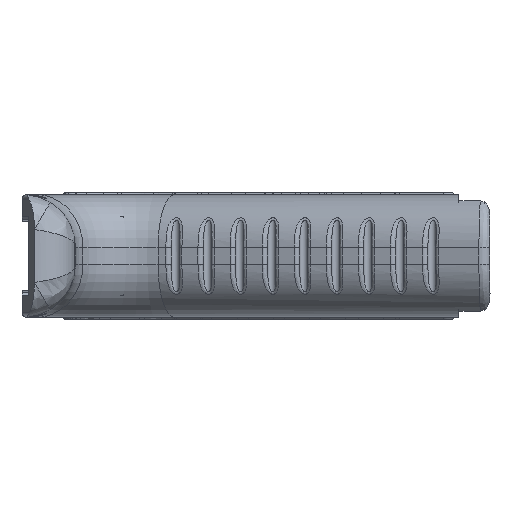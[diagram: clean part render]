
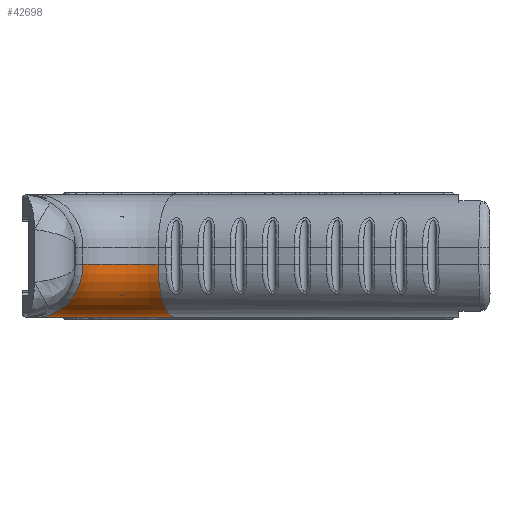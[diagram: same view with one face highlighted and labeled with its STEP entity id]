
A CAD part, left-side view. The second image highlights one B-rep face of the part: STEP entity #42698.
In plain terms, the highlighted toroidal (fillet/blend) face has major radius 27.537 mm and minor radius 12.5 mm.
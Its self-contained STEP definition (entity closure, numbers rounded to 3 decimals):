
#1002=TOROIDAL_SURFACE('',#44390,27.537,12.5);
#1278=B_SPLINE_CURVE_WITH_KNOTS('',3,(#81978,#81979,#81980,#81981,#81982,
#81983,#81984,#81985,#81986,#81987,#81988,#81989,#81990,#81991,#81992,#81993,
#81994,#81995,#81996,#81997,#81998,#81999,#82000,#82001,#82002,#82003,#82004,
#82005,#82006,#82007,#82008,#82009,#82010,#82011,#82012,#82013,#82014,#82015,
#82016,#82017,#82018,#82019,#82020,#82021,#82022,#82023,#82024,#82025,#82026,
#82027,#82028,#82029),.UNSPECIFIED.,.F.,.F.,(4,3,3,3,3,3,3,3,3,3,3,3,3,
3,3,3,3,4),(-0.008,0.,0.131,0.314,
0.448,0.497,0.627,0.806,
0.94,0.985,1.115,1.294,1.429,
1.473,1.604,1.783,1.915,1.961),
 .UNSPECIFIED.);
#3668=CIRCLE('',#43090,27.537);
#3890=CIRCLE('',#44312,15.037);
#3922=CIRCLE('',#44391,12.5);
#6183=FACE_OUTER_BOUND('',#8610,.T.);
#8610=EDGE_LOOP('',(#37997,#37998,#37999,#38000));
#16500=VERTEX_POINT('',#52969);
#16501=VERTEX_POINT('',#52971);
#20166=VERTEX_POINT('',#80456);
#20168=VERTEX_POINT('',#81551);
#20689=EDGE_CURVE('',#16501,#16500,#3668,.T.);
#26236=EDGE_CURVE('',#20166,#20168,#3890,.T.);
#26347=EDGE_CURVE('',#16501,#20168,#1278,.T.);
#26348=EDGE_CURVE('',#20166,#16500,#3922,.T.);
#37997=ORIENTED_EDGE('',*,*,#20689,.T.);
#37998=ORIENTED_EDGE('',*,*,#26348,.F.);
#37999=ORIENTED_EDGE('',*,*,#26236,.T.);
#38000=ORIENTED_EDGE('',*,*,#26347,.F.);
#42698=ADVANCED_FACE('',(#6183),#1002,.T.);
#43090=AXIS2_PLACEMENT_3D('',#52972,#45144,#45145);
#44312=AXIS2_PLACEMENT_3D('',#81552,#50798,#50799);
#44390=AXIS2_PLACEMENT_3D('',#82030,#51021,#51022);
#44391=AXIS2_PLACEMENT_3D('',#82031,#51023,#51024);
#45144=DIRECTION('center_axis',(0.,0.,-1.));
#45145=DIRECTION('ref_axis',(0.93,0.368,0.));
#50798=DIRECTION('center_axis',(0.,0.,1.));
#50799=DIRECTION('ref_axis',(0.93,0.368,0.));
#51021=DIRECTION('center_axis',(0.,0.,1.));
#51022=DIRECTION('ref_axis',(1.,0.,0.));
#51023=DIRECTION('center_axis',(-0.309,-0.951,0.));
#51024=DIRECTION('ref_axis',(-0.951,0.309,0.));
#52969=CARTESIAN_POINT('',(-54.134,133.337,-34.));
#52971=CARTESIAN_POINT('',(-66.871,165.874,-34.));
#52972=CARTESIAN_POINT('Origin',(-80.324,141.847,-34.));
#80456=CARTESIAN_POINT('',(-66.022,137.2,-21.5));
#81551=CARTESIAN_POINT('',(-73.077,155.023,-21.5));
#81552=CARTESIAN_POINT('Origin',(-80.324,141.847,-21.5));
#81978=CARTESIAN_POINT('Ctrl Pts',(-66.871,165.874,-34.));
#81979=CARTESIAN_POINT('Ctrl Pts',(-66.885,165.85,-34.));
#81980=CARTESIAN_POINT('Ctrl Pts',(-66.899,165.826,-34.));
#81981=CARTESIAN_POINT('Ctrl Pts',(-66.912,165.802,-34.));
#81982=CARTESIAN_POINT('Ctrl Pts',(-67.129,165.424,-33.997));
#81983=CARTESIAN_POINT('Ctrl Pts',(-67.344,165.047,-33.971));
#81984=CARTESIAN_POINT('Ctrl Pts',(-67.559,164.672,-33.923));
#81985=CARTESIAN_POINT('Ctrl Pts',(-67.858,164.148,-33.856));
#81986=CARTESIAN_POINT('Ctrl Pts',(-68.155,163.629,-33.745));
#81987=CARTESIAN_POINT('Ctrl Pts',(-68.446,163.119,-33.59));
#81988=CARTESIAN_POINT('Ctrl Pts',(-68.661,162.744,-33.477));
#81989=CARTESIAN_POINT('Ctrl Pts',(-68.873,162.374,-33.34));
#81990=CARTESIAN_POINT('Ctrl Pts',(-69.08,162.01,-33.181));
#81991=CARTESIAN_POINT('Ctrl Pts',(-69.155,161.88,-33.124));
#81992=CARTESIAN_POINT('Ctrl Pts',(-69.229,161.751,-33.064));
#81993=CARTESIAN_POINT('Ctrl Pts',(-69.302,161.622,-33.001));
#81994=CARTESIAN_POINT('Ctrl Pts',(-69.501,161.275,-32.83));
#81995=CARTESIAN_POINT('Ctrl Pts',(-69.695,160.936,-32.639));
#81996=CARTESIAN_POINT('Ctrl Pts',(-69.883,160.607,-32.429));
#81997=CARTESIAN_POINT('Ctrl Pts',(-70.141,160.156,-32.14));
#81998=CARTESIAN_POINT('Ctrl Pts',(-70.388,159.724,-31.815));
#81999=CARTESIAN_POINT('Ctrl Pts',(-70.623,159.313,-31.456));
#82000=CARTESIAN_POINT('Ctrl Pts',(-70.799,159.005,-31.187));
#82001=CARTESIAN_POINT('Ctrl Pts',(-70.969,158.709,-30.898));
#82002=CARTESIAN_POINT('Ctrl Pts',(-71.13,158.427,-30.591));
#82003=CARTESIAN_POINT('Ctrl Pts',(-71.184,158.333,-30.489));
#82004=CARTESIAN_POINT('Ctrl Pts',(-71.236,158.241,-30.386));
#82005=CARTESIAN_POINT('Ctrl Pts',(-71.288,158.15,-30.28));
#82006=CARTESIAN_POINT('Ctrl Pts',(-71.44,157.885,-29.971));
#82007=CARTESIAN_POINT('Ctrl Pts',(-71.583,157.635,-29.646));
#82008=CARTESIAN_POINT('Ctrl Pts',(-71.717,157.4,-29.308));
#82009=CARTESIAN_POINT('Ctrl Pts',(-71.901,157.078,-28.844));
#82010=CARTESIAN_POINT('Ctrl Pts',(-72.069,156.785,-28.354));
#82011=CARTESIAN_POINT('Ctrl Pts',(-72.219,156.523,-27.842));
#82012=CARTESIAN_POINT('Ctrl Pts',(-72.332,156.326,-27.456));
#82013=CARTESIAN_POINT('Ctrl Pts',(-72.435,156.146,-27.057));
#82014=CARTESIAN_POINT('Ctrl Pts',(-72.527,155.985,-26.647));
#82015=CARTESIAN_POINT('Ctrl Pts',(-72.556,155.933,-26.514));
#82016=CARTESIAN_POINT('Ctrl Pts',(-72.585,155.883,-26.38));
#82017=CARTESIAN_POINT('Ctrl Pts',(-72.613,155.835,-26.245));
#82018=CARTESIAN_POINT('Ctrl Pts',(-72.695,155.691,-25.841));
#82019=CARTESIAN_POINT('Ctrl Pts',(-72.767,155.566,-25.429));
#82020=CARTESIAN_POINT('Ctrl Pts',(-72.827,155.46,-25.012));
#82021=CARTESIAN_POINT('Ctrl Pts',(-72.91,155.315,-24.443));
#82022=CARTESIAN_POINT('Ctrl Pts',(-72.973,155.206,-23.862));
#82023=CARTESIAN_POINT('Ctrl Pts',(-73.014,155.133,-23.276));
#82024=CARTESIAN_POINT('Ctrl Pts',(-73.045,155.079,-22.84));
#82025=CARTESIAN_POINT('Ctrl Pts',(-73.065,155.044,-22.402));
#82026=CARTESIAN_POINT('Ctrl Pts',(-73.073,155.03,-21.961));
#82027=CARTESIAN_POINT('Ctrl Pts',(-73.076,155.025,-21.808));
#82028=CARTESIAN_POINT('Ctrl Pts',(-73.077,155.023,-21.654));
#82029=CARTESIAN_POINT('Ctrl Pts',(-73.077,155.023,-21.5));
#82030=CARTESIAN_POINT('Origin',(-80.324,141.847,-21.5));
#82031=CARTESIAN_POINT('Origin',(-54.134,133.337,-21.5));
